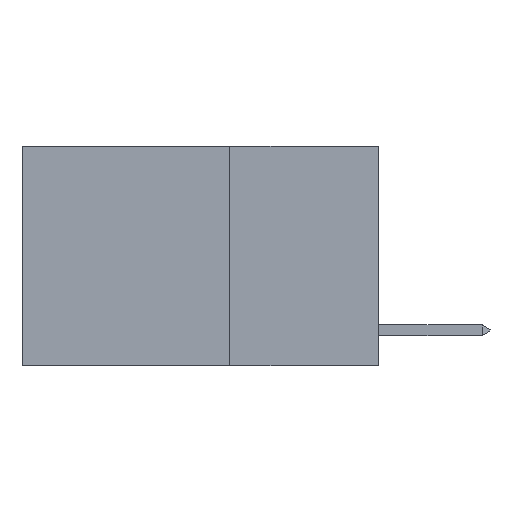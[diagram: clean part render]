
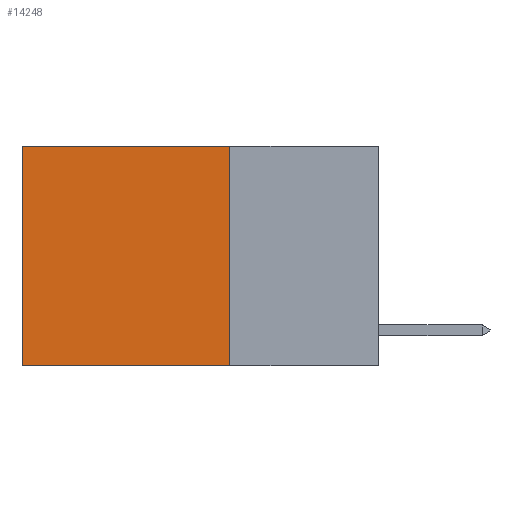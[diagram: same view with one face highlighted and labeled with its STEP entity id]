
A CAD part, left-side view. The second image highlights one B-rep face of the part: STEP entity #14248.
In plain terms, the highlighted planar face has unit normal (-1, 0, 0).
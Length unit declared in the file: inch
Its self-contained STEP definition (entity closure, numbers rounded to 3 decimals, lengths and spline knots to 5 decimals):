
#300 = DIRECTION ( 'NONE',  ( 1., 0., 0. ) ) ;
#678 = ORIENTED_EDGE ( 'NONE', *, *, #7165, .T. ) ;
#1526 = EDGE_CURVE ( 'NONE', #2421, #4072, #2373, .T. ) ;
#1785 = EDGE_LOOP ( 'NONE', ( #14554, #15339, #3064, #678 ) ) ;
#2373 = LINE ( 'NONE', #12528, #5866 ) ;
#2421 = VERTEX_POINT ( 'NONE', #10712 ) ;
#2817 = EDGE_CURVE ( 'NONE', #8418, #4072, #2907, .T. ) ;
#2907 = LINE ( 'NONE', #6325, #6424 ) ;
#3064 = ORIENTED_EDGE ( 'NONE', *, *, #5447, .F. ) ;
#4072 = VERTEX_POINT ( 'NONE', #7538 ) ;
#4277 = FACE_OUTER_BOUND ( 'NONE', #1785, .T. ) ;
#5001 = CARTESIAN_POINT ( 'NONE',  ( 0.2625, 0.25, 0. ) ) ;
#5447 = EDGE_CURVE ( 'NONE', #6582, #2421, #12395, .T. ) ;
#5723 = LINE ( 'NONE', #7745, #15283 ) ;
#5866 = VECTOR ( 'NONE', #9953, 39.37008 ) ;
#6325 = CARTESIAN_POINT ( 'NONE',  ( 0.2625, 0.6, 0. ) ) ;
#6424 = VECTOR ( 'NONE', #12780, 39.37008 ) ;
#6582 = VERTEX_POINT ( 'NONE', #5001 ) ;
#7165 = EDGE_CURVE ( 'NONE', #6582, #8418, #5723, .T. ) ;
#7538 = CARTESIAN_POINT ( 'NONE',  ( 0.2625, 0.6, -0.37 ) ) ;
#7745 = CARTESIAN_POINT ( 'NONE',  ( 0.2625, 0.25, 0. ) ) ;
#8418 = VERTEX_POINT ( 'NONE', #9774 ) ;
#8958 = VECTOR ( 'NONE', #10698, 39.37008 ) ;
#9534 = DIRECTION ( 'NONE',  ( 0., 0., -1. ) ) ;
#9774 = CARTESIAN_POINT ( 'NONE',  ( 0.2625, 0.6, 0. ) ) ;
#9953 = DIRECTION ( 'NONE',  ( 0., 1., 0. ) ) ;
#10698 = DIRECTION ( 'NONE',  ( 0., 0., -1. ) ) ;
#10712 = CARTESIAN_POINT ( 'NONE',  ( 0.2625, 0.25, -0.37 ) ) ;
#12203 = AXIS2_PLACEMENT_3D ( 'NONE', #15951, #300, #9534 ) ;
#12395 = LINE ( 'NONE', #15872, #8958 ) ;
#12528 = CARTESIAN_POINT ( 'NONE',  ( 0.2625, 0.25, -0.37 ) ) ;
#12780 = DIRECTION ( 'NONE',  ( 0., 0., -1. ) ) ;
#12945 = DIRECTION ( 'NONE',  ( 0., 1., 0. ) ) ;
#13351 = PLANE ( 'NONE',  #12203 ) ;
#14248 = ADVANCED_FACE ( 'NONE', ( #4277 ), #13351, .F. ) ;
#14554 = ORIENTED_EDGE ( 'NONE', *, *, #2817, .T. ) ;
#15283 = VECTOR ( 'NONE', #12945, 39.37008 ) ;
#15339 = ORIENTED_EDGE ( 'NONE', *, *, #1526, .F. ) ;
#15872 = CARTESIAN_POINT ( 'NONE',  ( 0.2625, 0.25, 0. ) ) ;
#15951 = CARTESIAN_POINT ( 'NONE',  ( 0.2625, 0.25, 0. ) ) ;
